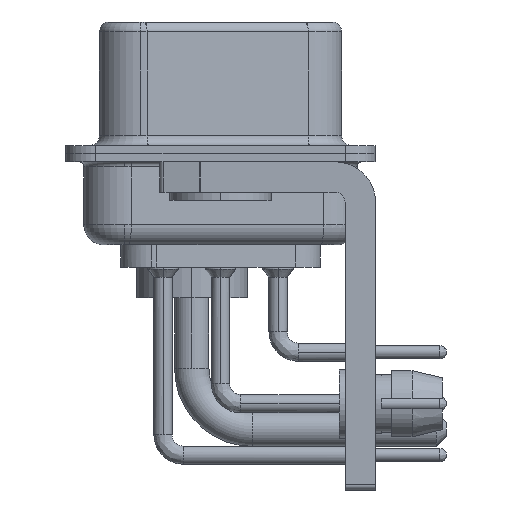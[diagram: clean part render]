
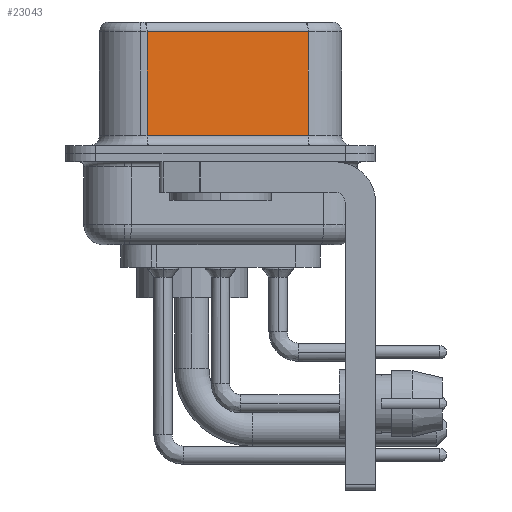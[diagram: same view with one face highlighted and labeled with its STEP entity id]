
A CAD part, left-side view. The second image highlights one B-rep face of the part: STEP entity #23043.
In plain terms, the highlighted planar face has unit normal (-0.985, -0.174, 0).
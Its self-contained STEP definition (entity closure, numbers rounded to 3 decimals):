
#1784 = EDGE_CURVE ( 'NONE', #17789, #29925, #36239, .T. ) ;
#3537 = FACE_OUTER_BOUND ( 'NONE', #23219, .T. ) ;
#4158 = EDGE_CURVE ( 'NONE', #29925, #32533, #27833, .T. ) ;
#5276 = ORIENTED_EDGE ( 'NONE', *, *, #4158, .T. ) ;
#6485 = VECTOR ( 'NONE', #36989, 1000. ) ;
#6725 = EDGE_CURVE ( 'NONE', #14254, #17789, #12006, .T. ) ;
#6824 = CARTESIAN_POINT ( 'NONE',  ( 5.132, -4.322, 6.02 ) ) ;
#8233 = ORIENTED_EDGE ( 'NONE', *, *, #1784, .T. ) ;
#8435 = CARTESIAN_POINT ( 'NONE',  ( 3.73, 3.628, 6.52 ) ) ;
#10108 = CARTESIAN_POINT ( 'NONE',  ( 5.132, -4.322, 0.9 ) ) ;
#10140 = VECTOR ( 'NONE', #22395, 1000. ) ;
#11224 = DIRECTION ( 'NONE',  ( 0., 0., -1. ) ) ;
#12006 = LINE ( 'NONE', #24496, #6485 ) ;
#14254 = VERTEX_POINT ( 'NONE', #6824 ) ;
#14604 = ORIENTED_EDGE ( 'NONE', *, *, #6725, .T. ) ;
#14966 = ORIENTED_EDGE ( 'NONE', *, *, #18780, .F. ) ;
#15601 = PLANE ( 'NONE',  #22286 ) ;
#17789 = VERTEX_POINT ( 'NONE', #36489 ) ;
#18780 = EDGE_CURVE ( 'NONE', #14254, #32533, #23902, .T. ) ;
#19738 = VECTOR ( 'NONE', #32419, 1000. ) ;
#20891 = CARTESIAN_POINT ( 'NONE',  ( 5.132, -4.322, 6.52 ) ) ;
#22286 = AXIS2_PLACEMENT_3D ( 'NONE', #22425, #28063, #24854 ) ;
#22395 = DIRECTION ( 'NONE',  ( 0.174, -0.985, 0. ) ) ;
#22425 = CARTESIAN_POINT ( 'NONE',  ( 5.132, -4.322, 6.52 ) ) ;
#23043 = ADVANCED_FACE ( 'NONE', ( #3537 ), #15601, .F. ) ;
#23219 = EDGE_LOOP ( 'NONE', ( #14966, #14604, #8233, #5276 ) ) ;
#23902 = LINE ( 'NONE', #20891, #27256 ) ;
#24496 = CARTESIAN_POINT ( 'NONE',  ( 5.132, -4.322, 6.02 ) ) ;
#24854 = DIRECTION ( 'NONE',  ( -0.174, 0.985, 0. ) ) ;
#27256 = VECTOR ( 'NONE', #11224, 1000. ) ;
#27833 = LINE ( 'NONE', #10108, #10140 ) ;
#28063 = DIRECTION ( 'NONE',  ( 0.985, 0.174, 0. ) ) ;
#29925 = VERTEX_POINT ( 'NONE', #38644 ) ;
#31649 = CARTESIAN_POINT ( 'NONE',  ( 5.132, -4.322, 0.9 ) ) ;
#32419 = DIRECTION ( 'NONE',  ( 0., 0., -1. ) ) ;
#32533 = VERTEX_POINT ( 'NONE', #31649 ) ;
#36239 = LINE ( 'NONE', #8435, #19738 ) ;
#36489 = CARTESIAN_POINT ( 'NONE',  ( 3.73, 3.628, 6.02 ) ) ;
#36989 = DIRECTION ( 'NONE',  ( -0.174, 0.985, 0. ) ) ;
#38644 = CARTESIAN_POINT ( 'NONE',  ( 3.73, 3.628, 0.9 ) ) ;
